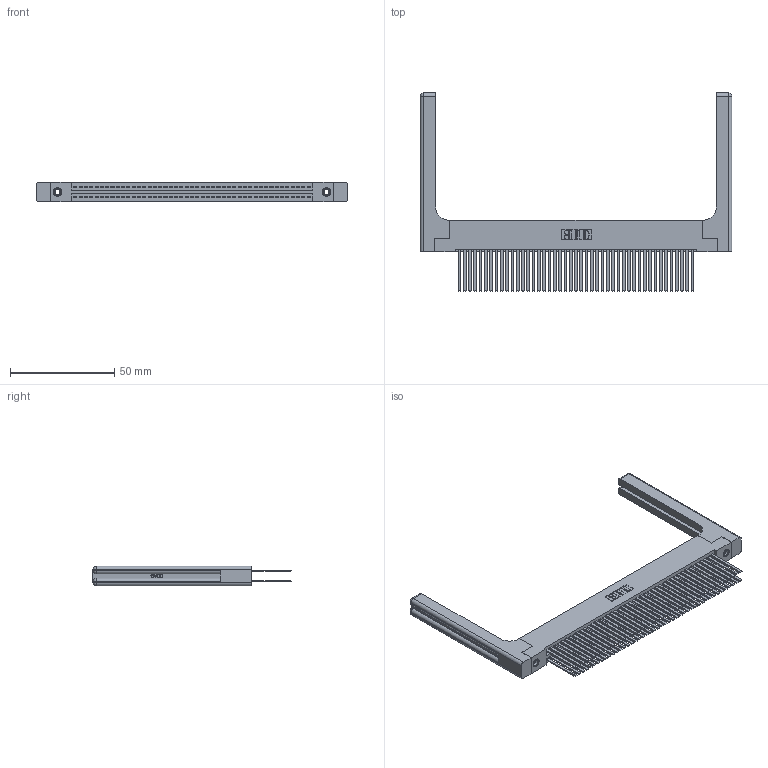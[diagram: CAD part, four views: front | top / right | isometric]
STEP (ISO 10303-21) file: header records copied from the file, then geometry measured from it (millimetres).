
FILE_DESCRIPTION (( 'STEP AP203' ), '1' );
FILE_NAME ('395-090-544-258.STEP', '2019-10-25T17:08:00', ( '' ), ( '' ), 'SwSTEP 2.0', 'SolidWorks 2016', '' );
FILE_SCHEMA (( 'CONFIG_CONTROL_DESIGN' ));
Length unit declared in the file: inch
Products named in the file (5): 395-090-544-258; 345 Part_Flush Mounting Lugs - 0.156 Dia-TH; 345-292-001_345-293-144; 345-250-001_345-250-001-102; 345-220-058_345-220-058
Assembly tree (95 placements, depth 2):
  395-090-544-258
    345 Part_Flush Mounting Lugs - 0.156 Dia-TH
    345-292-001_345-293-144  x90
    345-250-001_345-250-001-102  x2
    345-220-058_345-220-058  x2
Bounding box: 149.33 x 94.92 x 9.4 mm (x, y, z)
Volume: 24270.3 mm3; surface area: 32162.7 mm2
Topology: 95 solids, 95 shells, 4342 faces, 12797 edges, 8390 vertices
Faces by surface type: plane 2838, cylinder 1444, bspline 36, cone 12, sphere 8, torus 4
Entity records: 39902 total; most frequent: CARTESIAN_POINT 7677, ORIENTED_EDGE 6408, DIRECTION 5696, EDGE_CURVE 3204, VECTOR 2804, LINE 2804, VERTEX_POINT 2126, AXIS2_PLACEMENT_3D 1446
